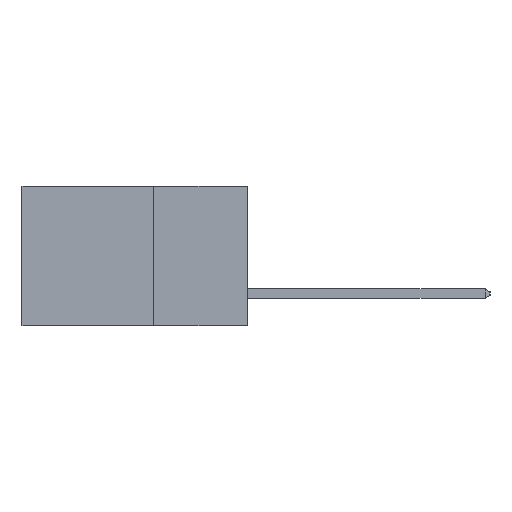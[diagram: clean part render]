
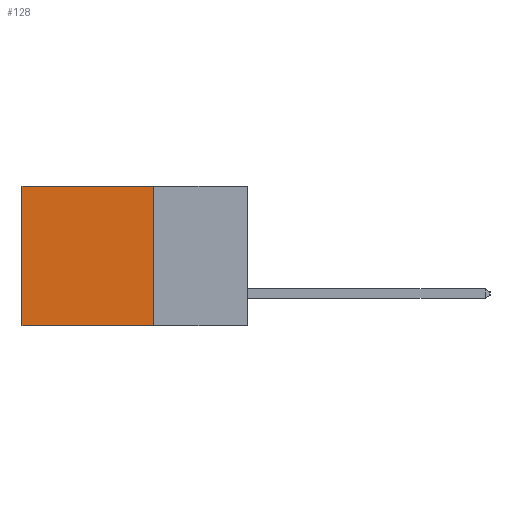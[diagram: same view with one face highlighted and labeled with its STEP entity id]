
A CAD part, left-side view. The second image highlights one B-rep face of the part: STEP entity #128.
In plain terms, the highlighted planar face has unit normal (-1, 0, 0).
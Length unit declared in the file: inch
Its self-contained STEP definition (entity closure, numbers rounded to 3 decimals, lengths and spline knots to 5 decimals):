
#128 = ADVANCED_FACE ( 'NONE', ( #7488 ), #16329, .F. ) ;
#630 = ORIENTED_EDGE ( 'NONE', *, *, #15074, .F. ) ;
#996 = VERTEX_POINT ( 'NONE', #16739 ) ;
#1318 = DIRECTION ( 'NONE',  ( 0., 0., -1. ) ) ;
#1391 = AXIS2_PLACEMENT_3D ( 'NONE', #8480, #9871, #1318 ) ;
#2283 = CARTESIAN_POINT ( 'NONE',  ( 0.2615, 0.6, 0. ) ) ;
#3573 = CARTESIAN_POINT ( 'NONE',  ( 0.2615, 0.6, -0.37 ) ) ;
#4412 = VECTOR ( 'NONE', #15695, 39.37008 ) ;
#5002 = LINE ( 'NONE', #3573, #15334 ) ;
#5016 = DIRECTION ( 'NONE',  ( 0., 0., -1. ) ) ;
#5382 = VERTEX_POINT ( 'NONE', #10010 ) ;
#6019 = VERTEX_POINT ( 'NONE', #2283 ) ;
#6401 = CARTESIAN_POINT ( 'NONE',  ( 0.2615, 0.25, -0.37 ) ) ;
#6515 = EDGE_CURVE ( 'NONE', #5382, #996, #7793, .T. ) ;
#6605 = EDGE_CURVE ( 'NONE', #5382, #6019, #9750, .T. ) ;
#7488 = FACE_OUTER_BOUND ( 'NONE', #8314, .T. ) ;
#7793 = LINE ( 'NONE', #7867, #4412 ) ;
#7838 = DIRECTION ( 'NONE',  ( 0., 1., 0. ) ) ;
#7867 = CARTESIAN_POINT ( 'NONE',  ( 0.2615, 0.25, -0.37 ) ) ;
#8099 = CARTESIAN_POINT ( 'NONE',  ( 0.2615, 0.25, 0. ) ) ;
#8314 = EDGE_LOOP ( 'NONE', ( #14809, #630, #10785, #16508 ) ) ;
#8480 = CARTESIAN_POINT ( 'NONE',  ( 0.2615, 0.25, -0.37 ) ) ;
#8622 = VECTOR ( 'NONE', #7838, 39.37008 ) ;
#9448 = CARTESIAN_POINT ( 'NONE',  ( 0.2615, 0.6, -0.37 ) ) ;
#9750 = LINE ( 'NONE', #8099, #12774 ) ;
#9871 = DIRECTION ( 'NONE',  ( 1., 0., 0. ) ) ;
#9873 = EDGE_CURVE ( 'NONE', #6019, #12756, #5002, .T. ) ;
#10010 = CARTESIAN_POINT ( 'NONE',  ( 0.2615, 0.25, 0. ) ) ;
#10785 = ORIENTED_EDGE ( 'NONE', *, *, #6515, .F. ) ;
#12131 = LINE ( 'NONE', #6401, #8622 ) ;
#12756 = VERTEX_POINT ( 'NONE', #9448 ) ;
#12774 = VECTOR ( 'NONE', #15974, 39.37008 ) ;
#14809 = ORIENTED_EDGE ( 'NONE', *, *, #9873, .T. ) ;
#15074 = EDGE_CURVE ( 'NONE', #996, #12756, #12131, .T. ) ;
#15334 = VECTOR ( 'NONE', #5016, 39.37008 ) ;
#15695 = DIRECTION ( 'NONE',  ( 0., 0., -1. ) ) ;
#15974 = DIRECTION ( 'NONE',  ( 0., 1., 0. ) ) ;
#16329 = PLANE ( 'NONE',  #1391 ) ;
#16508 = ORIENTED_EDGE ( 'NONE', *, *, #6605, .T. ) ;
#16739 = CARTESIAN_POINT ( 'NONE',  ( 0.2615, 0.25, -0.37 ) ) ;
